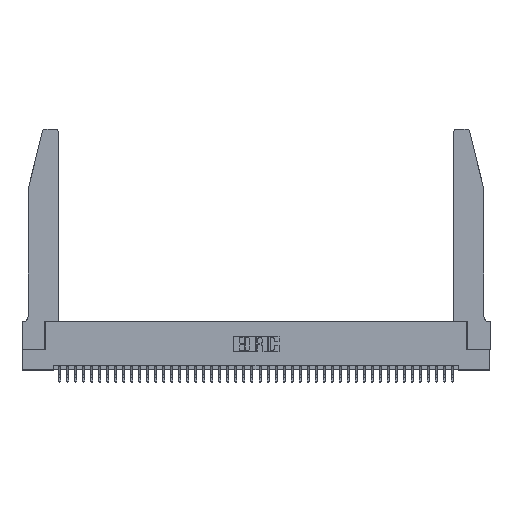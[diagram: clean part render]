
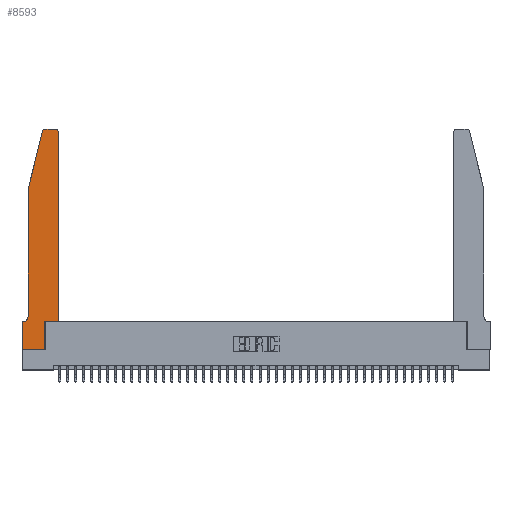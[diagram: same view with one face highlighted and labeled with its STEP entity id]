
A CAD part, top view. The second image highlights one B-rep face of the part: STEP entity #8593.
In plain terms, the highlighted planar face has unit normal (0, 0, 1).
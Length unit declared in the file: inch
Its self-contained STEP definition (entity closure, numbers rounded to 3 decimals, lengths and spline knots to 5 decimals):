
#488 = CARTESIAN_POINT ( 'NONE',  ( 0.4505, 2.72, 0.37 ) ) ;
#1534 = EDGE_CURVE ( 'NONE', #7830, #42834, #19651, .T. ) ;
#1915 = EDGE_CURVE ( 'NONE', #18074, #38847, #12876, .T. ) ;
#2002 = DIRECTION ( 'NONE',  ( -1., 0., 0. ) ) ;
#2066 = DIRECTION ( 'NONE',  ( 1., 0., 0. ) ) ;
#2130 = DIRECTION ( 'NONE',  ( -1., 0., 0. ) ) ;
#2566 = DIRECTION ( 'NONE',  ( 0., -1., 0. ) ) ;
#3088 = EDGE_CURVE ( 'NONE', #20636, #14928, #4927, .T. ) ;
#3726 = ORIENTED_EDGE ( 'NONE', *, *, #1534, .T. ) ;
#3866 = VECTOR ( 'NONE', #20996, 39.37008 ) ;
#3971 = LINE ( 'NONE', #40766, #29500 ) ;
#4927 = LINE ( 'NONE', #27372, #13855 ) ;
#6063 = ORIENTED_EDGE ( 'NONE', *, *, #6613, .T. ) ;
#6613 = EDGE_CURVE ( 'NONE', #17804, #41186, #41855, .T. ) ;
#7440 = ORIENTED_EDGE ( 'NONE', *, *, #1915, .T. ) ;
#7811 = LINE ( 'NONE', #40358, #33270 ) ;
#7830 = VERTEX_POINT ( 'NONE', #38099 ) ;
#7992 = VERTEX_POINT ( 'NONE', #32302 ) ;
#8593 = ADVANCED_FACE ( 'NONE', ( #29762 ), #25296, .T. ) ;
#8685 = VECTOR ( 'NONE', #2002, 39.37008 ) ;
#9896 = CARTESIAN_POINT ( 'NONE',  ( 0.2865, 0., 0.37 ) ) ;
#10656 = CIRCLE ( 'NONE', #31014, 0.03 ) ;
#10970 = DIRECTION ( 'NONE',  ( 0., 0., 1. ) ) ;
#10983 = CARTESIAN_POINT ( 'NONE',  ( 0.284, 2.72, 0.37 ) ) ;
#11295 = EDGE_CURVE ( 'NONE', #41186, #39139, #10656, .T. ) ;
#11903 = VECTOR ( 'NONE', #35182, 39.37008 ) ;
#12550 = CIRCLE ( 'NONE', #33299, 0.03 ) ;
#12876 = LINE ( 'NONE', #20843, #3866 ) ;
#13855 = VECTOR ( 'NONE', #20745, 39.37008 ) ;
#14314 = DIRECTION ( 'NONE',  ( 1., 0., 0. ) ) ;
#14320 = EDGE_CURVE ( 'NONE', #22747, #17804, #12550, .T. ) ;
#14734 = CARTESIAN_POINT ( 'NONE',  ( 0.0755, 2., 0.37 ) ) ;
#14928 = VERTEX_POINT ( 'NONE', #37274 ) ;
#15313 = CARTESIAN_POINT ( 'NONE',  ( 0.2865, 0.35, 0.37 ) ) ;
#16335 = EDGE_CURVE ( 'NONE', #42834, #20636, #19611, .T. ) ;
#17804 = VERTEX_POINT ( 'NONE', #29458 ) ;
#17921 = ORIENTED_EDGE ( 'NONE', *, *, #16335, .T. ) ;
#18074 = VERTEX_POINT ( 'NONE', #20782 ) ;
#18320 = CARTESIAN_POINT ( 'NONE',  ( 0.284, 2.75, 0.37 ) ) ;
#18680 = CARTESIAN_POINT ( 'NONE',  ( 0., 0., 0.37 ) ) ;
#18985 = ORIENTED_EDGE ( 'NONE', *, *, #3088, .T. ) ;
#19060 = AXIS2_PLACEMENT_3D ( 'NONE', #41921, #22108, #2066 ) ;
#19611 = LINE ( 'NONE', #15313, #28373 ) ;
#19651 = LINE ( 'NONE', #18680, #11903 ) ;
#20636 = VERTEX_POINT ( 'NONE', #30634 ) ;
#20745 = DIRECTION ( 'NONE',  ( 1., 0., 0. ) ) ;
#20782 = CARTESIAN_POINT ( 'NONE',  ( 0.0055, 0.35, 0.37 ) ) ;
#20843 = CARTESIAN_POINT ( 'NONE',  ( 0.0755, 0.35, 0.37 ) ) ;
#20996 = DIRECTION ( 'NONE',  ( -1., 0., 0. ) ) ;
#21379 = DIRECTION ( 'NONE',  ( -0.239, -0.971, 0. ) ) ;
#21882 = EDGE_CURVE ( 'NONE', #14928, #22747, #7811, .T. ) ;
#21966 = DIRECTION ( 'NONE',  ( 0., 1., 0. ) ) ;
#22046 = CARTESIAN_POINT ( 'NONE',  ( 0.2605, 2.75, 0.37 ) ) ;
#22108 = DIRECTION ( 'NONE',  ( 0., 0., 1. ) ) ;
#22170 = DIRECTION ( 'NONE',  ( 0., 0., -1. ) ) ;
#22607 = CARTESIAN_POINT ( 'NONE',  ( 0., 0., 0.37 ) ) ;
#22747 = VERTEX_POINT ( 'NONE', #488 ) ;
#23439 = CARTESIAN_POINT ( 'NONE',  ( 0.0755, 2., 0.37 ) ) ;
#24086 = ORIENTED_EDGE ( 'NONE', *, *, #36539, .T. ) ;
#24283 = DIRECTION ( 'NONE',  ( 0., -1., 0. ) ) ;
#24711 = LINE ( 'NONE', #22607, #41273 ) ;
#25183 = ORIENTED_EDGE ( 'NONE', *, *, #14320, .T. ) ;
#25266 = VERTEX_POINT ( 'NONE', #23439 ) ;
#25296 = PLANE ( 'NONE',  #19060 ) ;
#25366 = VECTOR ( 'NONE', #21379, 39.37008 ) ;
#27372 = CARTESIAN_POINT ( 'NONE',  ( 0.4505, 0.35, 0.37 ) ) ;
#28297 = CARTESIAN_POINT ( 'NONE',  ( 0.25487, 2.72718, 0.37 ) ) ;
#28373 = VECTOR ( 'NONE', #21966, 39.37008 ) ;
#29275 = ORIENTED_EDGE ( 'NONE', *, *, #34721, .T. ) ;
#29458 = CARTESIAN_POINT ( 'NONE',  ( 0.4205, 2.75, 0.37 ) ) ;
#29500 = VECTOR ( 'NONE', #24283, 39.37008 ) ;
#29762 = FACE_OUTER_BOUND ( 'NONE', #41485, .T. ) ;
#29807 = ORIENTED_EDGE ( 'NONE', *, *, #21882, .T. ) ;
#30537 = DIRECTION ( 'NONE',  ( 0., 1., 0. ) ) ;
#30593 = CIRCLE ( 'NONE', #32263, 0.07 ) ;
#30634 = CARTESIAN_POINT ( 'NONE',  ( 0.2865, 0.35, 0.37 ) ) ;
#30802 = CARTESIAN_POINT ( 'NONE',  ( 0.4205, 2.72, 0.37 ) ) ;
#31014 = AXIS2_PLACEMENT_3D ( 'NONE', #10983, #34173, #14314 ) ;
#32263 = AXIS2_PLACEMENT_3D ( 'NONE', #41980, #22170, #2130 ) ;
#32302 = CARTESIAN_POINT ( 'NONE',  ( 0.0755, 0.42, 0.37 ) ) ;
#33270 = VECTOR ( 'NONE', #30537, 39.37008 ) ;
#33299 = AXIS2_PLACEMENT_3D ( 'NONE', #30802, #10970, #34159 ) ;
#33620 = ORIENTED_EDGE ( 'NONE', *, *, #11295, .T. ) ;
#34159 = DIRECTION ( 'NONE',  ( 1., 0., 0. ) ) ;
#34168 = ORIENTED_EDGE ( 'NONE', *, *, #36967, .T. ) ;
#34173 = DIRECTION ( 'NONE',  ( 0., 0., 1. ) ) ;
#34206 = LINE ( 'NONE', #14734, #25366 ) ;
#34680 = ORIENTED_EDGE ( 'NONE', *, *, #42461, .T. ) ;
#34721 = EDGE_CURVE ( 'NONE', #38847, #7830, #24711, .T. ) ;
#35182 = DIRECTION ( 'NONE',  ( 1., 0., 0. ) ) ;
#36539 = EDGE_CURVE ( 'NONE', #7992, #18074, #30593, .T. ) ;
#36877 = CARTESIAN_POINT ( 'NONE',  ( 0., 0.35, 0.37 ) ) ;
#36967 = EDGE_CURVE ( 'NONE', #25266, #7992, #3971, .T. ) ;
#37274 = CARTESIAN_POINT ( 'NONE',  ( 0.4505, 0.35, 0.37 ) ) ;
#38099 = CARTESIAN_POINT ( 'NONE',  ( 0., 0., 0.37 ) ) ;
#38847 = VERTEX_POINT ( 'NONE', #36877 ) ;
#39139 = VERTEX_POINT ( 'NONE', #28297 ) ;
#40358 = CARTESIAN_POINT ( 'NONE',  ( 0.4505, 0.35, 0.37 ) ) ;
#40766 = CARTESIAN_POINT ( 'NONE',  ( 0.0755, 2., 0.37 ) ) ;
#41186 = VERTEX_POINT ( 'NONE', #18320 ) ;
#41273 = VECTOR ( 'NONE', #2566, 39.37008 ) ;
#41485 = EDGE_LOOP ( 'NONE', ( #6063, #33620, #34680, #34168, #24086, #7440, #29275, #3726, #17921, #18985, #29807, #25183 ) ) ;
#41855 = LINE ( 'NONE', #22046, #8685 ) ;
#41921 = CARTESIAN_POINT ( 'NONE',  ( 0., 0.35, 0.37 ) ) ;
#41980 = CARTESIAN_POINT ( 'NONE',  ( 0.0055, 0.42, 0.37 ) ) ;
#42461 = EDGE_CURVE ( 'NONE', #39139, #25266, #34206, .T. ) ;
#42834 = VERTEX_POINT ( 'NONE', #9896 ) ;
